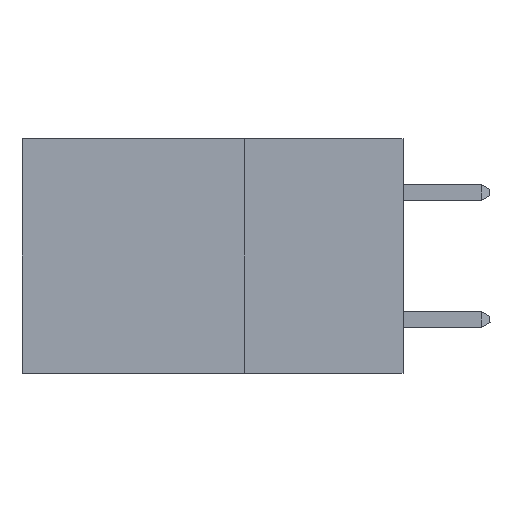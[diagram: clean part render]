
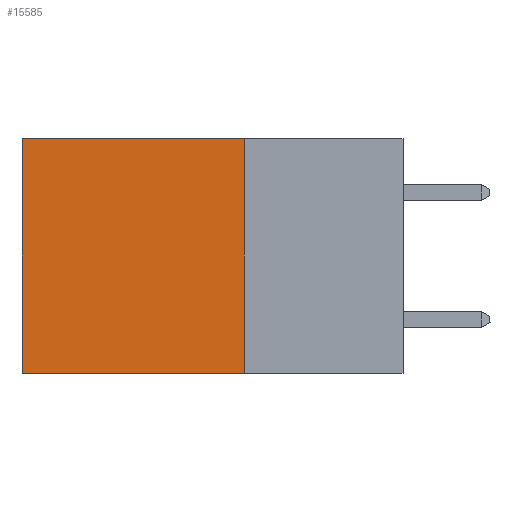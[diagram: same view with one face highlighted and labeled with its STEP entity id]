
A CAD part, left-side view. The second image highlights one B-rep face of the part: STEP entity #15585.
In plain terms, the highlighted planar face has unit normal (-1, 0, 0).
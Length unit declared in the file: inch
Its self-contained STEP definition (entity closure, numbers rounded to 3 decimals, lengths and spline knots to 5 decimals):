
#204 = EDGE_CURVE ( 'NONE', #18503, #16363, #19946, .T. ) ;
#351 = ORIENTED_EDGE ( 'NONE', *, *, #204, .F. ) ;
#403 = CARTESIAN_POINT ( 'NONE',  ( 0.2875, 0.25, 0. ) ) ;
#502 = CARTESIAN_POINT ( 'NONE',  ( 0.2875, 0.25, -0.37 ) ) ;
#1032 = CARTESIAN_POINT ( 'NONE',  ( 0.2875, 0.6, 0. ) ) ;
#1545 = DIRECTION ( 'NONE',  ( 1., 0., 0. ) ) ;
#1627 = CARTESIAN_POINT ( 'NONE',  ( 0.2875, 0.6, -0.37 ) ) ;
#1908 = EDGE_CURVE ( 'NONE', #1953, #16363, #20531, .T. ) ;
#1953 = VERTEX_POINT ( 'NONE', #17415 ) ;
#2245 = DIRECTION ( 'NONE',  ( 0., 0., -1. ) ) ;
#2625 = CARTESIAN_POINT ( 'NONE',  ( 0.2875, 0.25, 0. ) ) ;
#2752 = DIRECTION ( 'NONE',  ( 0., 0., -1. ) ) ;
#2950 = PLANE ( 'NONE',  #12048 ) ;
#3128 = ORIENTED_EDGE ( 'NONE', *, *, #17167, .T. ) ;
#3213 = LINE ( 'NONE', #2625, #15108 ) ;
#5177 = DIRECTION ( 'NONE',  ( 0., 1., 0. ) ) ;
#5448 = VECTOR ( 'NONE', #2752, 39.37008 ) ;
#5598 = VERTEX_POINT ( 'NONE', #8421 ) ;
#7845 = CARTESIAN_POINT ( 'NONE',  ( 0.2875, 0.25, -0.37 ) ) ;
#8421 = CARTESIAN_POINT ( 'NONE',  ( 0.2875, 0.25, 0. ) ) ;
#8710 = ORIENTED_EDGE ( 'NONE', *, *, #1908, .T. ) ;
#9783 = LINE ( 'NONE', #403, #10290 ) ;
#10290 = VECTOR ( 'NONE', #5177, 39.37008 ) ;
#10935 = VECTOR ( 'NONE', #20713, 39.37008 ) ;
#12048 = AXIS2_PLACEMENT_3D ( 'NONE', #13481, #1545, #2245 ) ;
#12149 = FACE_OUTER_BOUND ( 'NONE', #18931, .T. ) ;
#12195 = ORIENTED_EDGE ( 'NONE', *, *, #19872, .F. ) ;
#13481 = CARTESIAN_POINT ( 'NONE',  ( 0.2875, 0.25, 0. ) ) ;
#14465 = DIRECTION ( 'NONE',  ( 0., 0., -1. ) ) ;
#15108 = VECTOR ( 'NONE', #14465, 39.37008 ) ;
#15585 = ADVANCED_FACE ( 'NONE', ( #12149 ), #2950, .F. ) ;
#16363 = VERTEX_POINT ( 'NONE', #1627 ) ;
#17167 = EDGE_CURVE ( 'NONE', #5598, #1953, #9783, .T. ) ;
#17415 = CARTESIAN_POINT ( 'NONE',  ( 0.2875, 0.6, 0. ) ) ;
#18503 = VERTEX_POINT ( 'NONE', #7845 ) ;
#18931 = EDGE_LOOP ( 'NONE', ( #8710, #351, #12195, #3128 ) ) ;
#19872 = EDGE_CURVE ( 'NONE', #5598, #18503, #3213, .T. ) ;
#19946 = LINE ( 'NONE', #502, #10935 ) ;
#20531 = LINE ( 'NONE', #1032, #5448 ) ;
#20713 = DIRECTION ( 'NONE',  ( 0., 1., 0. ) ) ;
